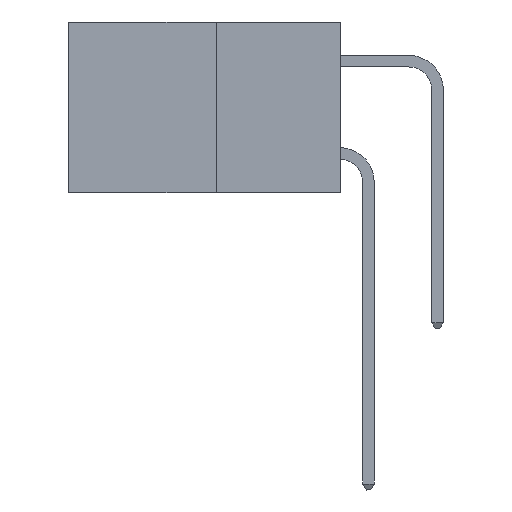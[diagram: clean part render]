
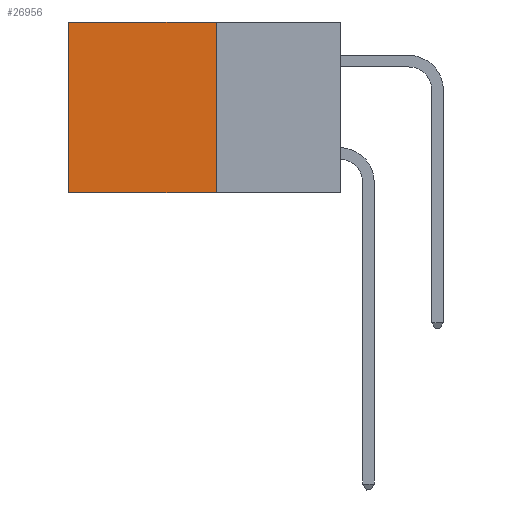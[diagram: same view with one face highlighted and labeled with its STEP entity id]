
A CAD part, left-side view. The second image highlights one B-rep face of the part: STEP entity #26956.
In plain terms, the highlighted planar face has unit normal (-1, 0, 0).
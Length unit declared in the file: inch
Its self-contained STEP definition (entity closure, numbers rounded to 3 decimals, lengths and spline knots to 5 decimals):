
#104 = EDGE_CURVE ( 'NONE', #24356, #30584, #17786, .T. ) ;
#1239 = VECTOR ( 'NONE', #5547, 39.37008 ) ;
#2124 = LINE ( 'NONE', #8235, #1239 ) ;
#4121 = CARTESIAN_POINT ( 'NONE',  ( 0.277, 0.59, 0. ) ) ;
#4175 = DIRECTION ( 'NONE',  ( 0., 1., 0. ) ) ;
#5058 = CARTESIAN_POINT ( 'NONE',  ( 0.277, 0.27, 0. ) ) ;
#5134 = CARTESIAN_POINT ( 'NONE',  ( 0.277, 0.27, 0. ) ) ;
#5547 = DIRECTION ( 'NONE',  ( 0., 0., -1. ) ) ;
#6163 = VERTEX_POINT ( 'NONE', #5134 ) ;
#7631 = CARTESIAN_POINT ( 'NONE',  ( 0.277, 0.59, -0.37 ) ) ;
#8078 = VERTEX_POINT ( 'NONE', #15053 ) ;
#8235 = CARTESIAN_POINT ( 'NONE',  ( 0.277, 0.27, -0.37 ) ) ;
#8623 = EDGE_CURVE ( 'NONE', #8078, #30584, #26548, .T. ) ;
#9580 = EDGE_CURVE ( 'NONE', #6163, #24356, #10519, .T. ) ;
#10312 = ORIENTED_EDGE ( 'NONE', *, *, #104, .T. ) ;
#10519 = LINE ( 'NONE', #5058, #30931 ) ;
#11055 = DIRECTION ( 'NONE',  ( 1., 0., 0. ) ) ;
#11814 = EDGE_CURVE ( 'NONE', #6163, #8078, #2124, .T. ) ;
#12254 = DIRECTION ( 'NONE',  ( 0., 0., -1. ) ) ;
#13874 = EDGE_LOOP ( 'NONE', ( #10312, #23591, #24151, #22802 ) ) ;
#14012 = VECTOR ( 'NONE', #4175, 39.37008 ) ;
#15053 = CARTESIAN_POINT ( 'NONE',  ( 0.277, 0.27, -0.37 ) ) ;
#16771 = FACE_OUTER_BOUND ( 'NONE', #13874, .T. ) ;
#17199 = CARTESIAN_POINT ( 'NONE',  ( 0.277, 0.59, -0.37 ) ) ;
#17786 = LINE ( 'NONE', #7631, #18650 ) ;
#18650 = VECTOR ( 'NONE', #12254, 39.37008 ) ;
#20583 = CARTESIAN_POINT ( 'NONE',  ( 0.277, 0.27, -0.37 ) ) ;
#21612 = AXIS2_PLACEMENT_3D ( 'NONE', #21631, #11055, #29706 ) ;
#21631 = CARTESIAN_POINT ( 'NONE',  ( 0.277, 0.27, -0.37 ) ) ;
#22802 = ORIENTED_EDGE ( 'NONE', *, *, #9580, .T. ) ;
#23591 = ORIENTED_EDGE ( 'NONE', *, *, #8623, .F. ) ;
#24151 = ORIENTED_EDGE ( 'NONE', *, *, #11814, .F. ) ;
#24356 = VERTEX_POINT ( 'NONE', #4121 ) ;
#26548 = LINE ( 'NONE', #20583, #14012 ) ;
#26956 = ADVANCED_FACE ( 'NONE', ( #16771 ), #27090, .F. ) ;
#27090 = PLANE ( 'NONE',  #21612 ) ;
#29250 = DIRECTION ( 'NONE',  ( 0., 1., 0. ) ) ;
#29706 = DIRECTION ( 'NONE',  ( 0., 0., -1. ) ) ;
#30584 = VERTEX_POINT ( 'NONE', #17199 ) ;
#30931 = VECTOR ( 'NONE', #29250, 39.37008 ) ;
